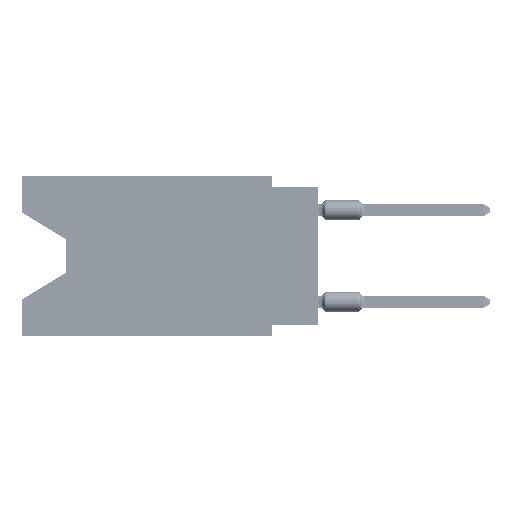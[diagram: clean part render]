
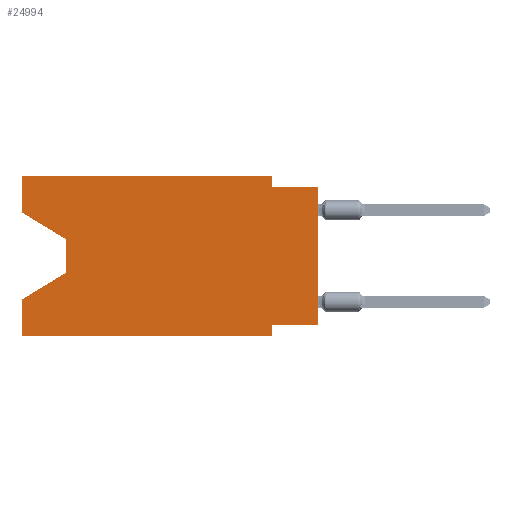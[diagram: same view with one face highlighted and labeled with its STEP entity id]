
A CAD part, left-side view. The second image highlights one B-rep face of the part: STEP entity #24994.
In plain terms, the highlighted planar face has unit normal (-1, 0, 0).
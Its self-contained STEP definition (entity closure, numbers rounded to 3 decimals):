
#139 = LINE ( 'NONE', #114180, #81911 ) ;
#1110 = EDGE_CURVE ( 'NONE', #107210, #41197, #100415, .T. ) ;
#3714 = DIRECTION ( 'NONE',  ( 0., 0.855, -0.519 ) ) ;
#4811 = CARTESIAN_POINT ( 'NONE',  ( 0., 16.383, 0. ) ) ;
#5050 = EDGE_LOOP ( 'NONE', ( #55344, #67228, #28012, #42846, #88379, #29049, #16364, #54764, #113163, #54858, #100345, #48149 ) ) ;
#8114 = CARTESIAN_POINT ( 'NONE',  ( 0., 13.97, -3.505 ) ) ;
#8500 = CARTESIAN_POINT ( 'NONE',  ( 0., 16.383, 0. ) ) ;
#9137 = VECTOR ( 'NONE', #3714, 1000. ) ;
#10500 = VERTEX_POINT ( 'NONE', #104164 ) ;
#11491 = EDGE_CURVE ( 'NONE', #29084, #54442, #13577, .T. ) ;
#11875 = LINE ( 'NONE', #30008, #97295 ) ;
#12349 = CARTESIAN_POINT ( 'NONE',  ( 0., 16.383, 0. ) ) ;
#12942 = CARTESIAN_POINT ( 'NONE',  ( 0., 13.97, -3.505 ) ) ;
#13577 = LINE ( 'NONE', #56252, #45236 ) ;
#14923 = CARTESIAN_POINT ( 'NONE',  ( 0., 16.383, -6.852 ) ) ;
#15691 = CARTESIAN_POINT ( 'NONE',  ( 0., 0., -8.255 ) ) ;
#16031 = VECTOR ( 'NONE', #113544, 1000. ) ;
#16187 = VERTEX_POINT ( 'NONE', #26955 ) ;
#16364 = ORIENTED_EDGE ( 'NONE', *, *, #80838, .F. ) ;
#17257 = EDGE_CURVE ( 'NONE', #10500, #16187, #61457, .T. ) ;
#18550 = VECTOR ( 'NONE', #60354, 1000. ) ;
#19495 = VECTOR ( 'NONE', #22275, 1000. ) ;
#20193 = FACE_OUTER_BOUND ( 'NONE', #5050, .T. ) ;
#20897 = CARTESIAN_POINT ( 'NONE',  ( 0., 16.383, -2.038 ) ) ;
#22275 = DIRECTION ( 'NONE',  ( 0., 0., 1. ) ) ;
#24994 = ADVANCED_FACE ( 'NONE', ( #20193 ), #84902, .F. ) ;
#25699 = VERTEX_POINT ( 'NONE', #15691 ) ;
#25888 = LINE ( 'NONE', #114182, #18550 ) ;
#26062 = LINE ( 'NONE', #8500, #71892 ) ;
#26821 = CARTESIAN_POINT ( 'NONE',  ( 0., 13.97, -5.385 ) ) ;
#26955 = CARTESIAN_POINT ( 'NONE',  ( 0., 2.54, -0.635 ) ) ;
#28012 = ORIENTED_EDGE ( 'NONE', *, *, #89920, .T. ) ;
#29049 = ORIENTED_EDGE ( 'NONE', *, *, #91329, .F. ) ;
#29084 = VERTEX_POINT ( 'NONE', #59069 ) ;
#30008 = CARTESIAN_POINT ( 'NONE',  ( 0., 0., -8.255 ) ) ;
#30489 = LINE ( 'NONE', #12349, #19495 ) ;
#31636 = LINE ( 'NONE', #111734, #78249 ) ;
#31715 = DIRECTION ( 'NONE',  ( 0., -1., 0. ) ) ;
#32287 = DIRECTION ( 'NONE',  ( 0., 0., -1. ) ) ;
#32775 = DIRECTION ( 'NONE',  ( 0., 0., 1. ) ) ;
#35383 = DIRECTION ( 'NONE',  ( 0., -1., 0. ) ) ;
#35418 = VECTOR ( 'NONE', #42100, 1000. ) ;
#35787 = DIRECTION ( 'NONE',  ( 0., 0., -1. ) ) ;
#35886 = VERTEX_POINT ( 'NONE', #73316 ) ;
#38751 = DIRECTION ( 'NONE',  ( 0., 1., 0. ) ) ;
#41197 = VERTEX_POINT ( 'NONE', #12942 ) ;
#42100 = DIRECTION ( 'NONE',  ( 0., -1., 0. ) ) ;
#42197 = CARTESIAN_POINT ( 'NONE',  ( 0., 2.54, 0. ) ) ;
#42846 = ORIENTED_EDGE ( 'NONE', *, *, #70744, .F. ) ;
#45236 = VECTOR ( 'NONE', #31715, 1000. ) ;
#48149 = ORIENTED_EDGE ( 'NONE', *, *, #78476, .F. ) ;
#51134 = CARTESIAN_POINT ( 'NONE',  ( 0., 16.383, 0. ) ) ;
#51431 = LINE ( 'NONE', #87700, #35418 ) ;
#51516 = DIRECTION ( 'NONE',  ( 1., 0., 0. ) ) ;
#54442 = VERTEX_POINT ( 'NONE', #76331 ) ;
#54764 = ORIENTED_EDGE ( 'NONE', *, *, #61824, .T. ) ;
#54858 = ORIENTED_EDGE ( 'NONE', *, *, #17257, .F. ) ;
#55344 = ORIENTED_EDGE ( 'NONE', *, *, #1110, .T. ) ;
#55789 = EDGE_CURVE ( 'NONE', #72220, #10500, #26062, .T. ) ;
#56252 = CARTESIAN_POINT ( 'NONE',  ( 0., 16.383, -8.89 ) ) ;
#59069 = CARTESIAN_POINT ( 'NONE',  ( 0., 16.383, -8.89 ) ) ;
#60354 = DIRECTION ( 'NONE',  ( 0., 0., 1. ) ) ;
#61457 = LINE ( 'NONE', #42197, #16031 ) ;
#61824 = EDGE_CURVE ( 'NONE', #25699, #35886, #25888, .T. ) ;
#64222 = VECTOR ( 'NONE', #115104, 1000. ) ;
#64727 = DIRECTION ( 'NONE',  ( 0., -0.855, -0.519 ) ) ;
#66817 = LINE ( 'NONE', #92572, #9137 ) ;
#67228 = ORIENTED_EDGE ( 'NONE', *, *, #101912, .T. ) ;
#67955 = CARTESIAN_POINT ( 'NONE',  ( 0., 16.383, -2.038 ) ) ;
#70744 = EDGE_CURVE ( 'NONE', #29084, #108419, #31636, .T. ) ;
#71892 = VECTOR ( 'NONE', #35383, 1000. ) ;
#72220 = VERTEX_POINT ( 'NONE', #51134 ) ;
#73077 = EDGE_CURVE ( 'NONE', #16187, #35886, #51431, .T. ) ;
#73316 = CARTESIAN_POINT ( 'NONE',  ( 0., 0., -0.635 ) ) ;
#73793 = VECTOR ( 'NONE', #64727, 1000. ) ;
#76331 = CARTESIAN_POINT ( 'NONE',  ( 0., 2.54, -8.89 ) ) ;
#78249 = VECTOR ( 'NONE', #32775, 1000. ) ;
#78476 = EDGE_CURVE ( 'NONE', #107210, #72220, #30489, .T. ) ;
#80838 = EDGE_CURVE ( 'NONE', #25699, #95341, #11875, .T. ) ;
#81911 = VECTOR ( 'NONE', #35787, 1000. ) ;
#84902 = PLANE ( 'NONE',  #106327 ) ;
#87700 = CARTESIAN_POINT ( 'NONE',  ( 0., 0., -0.635 ) ) ;
#88379 = ORIENTED_EDGE ( 'NONE', *, *, #11491, .T. ) ;
#89920 = EDGE_CURVE ( 'NONE', #102997, #108419, #66817, .T. ) ;
#91329 = EDGE_CURVE ( 'NONE', #95341, #54442, #139, .T. ) ;
#92572 = CARTESIAN_POINT ( 'NONE',  ( 0., 13.97, -5.385 ) ) ;
#95341 = VERTEX_POINT ( 'NONE', #114263 ) ;
#97295 = VECTOR ( 'NONE', #38751, 1000. ) ;
#100345 = ORIENTED_EDGE ( 'NONE', *, *, #55789, .F. ) ;
#100415 = LINE ( 'NONE', #20897, #73793 ) ;
#101912 = EDGE_CURVE ( 'NONE', #41197, #102997, #106324, .T. ) ;
#102997 = VERTEX_POINT ( 'NONE', #26821 ) ;
#104164 = CARTESIAN_POINT ( 'NONE',  ( 0., 2.54, 0. ) ) ;
#106324 = LINE ( 'NONE', #8114, #64222 ) ;
#106327 = AXIS2_PLACEMENT_3D ( 'NONE', #4811, #51516, #32287 ) ;
#107210 = VERTEX_POINT ( 'NONE', #67955 ) ;
#108419 = VERTEX_POINT ( 'NONE', #14923 ) ;
#111734 = CARTESIAN_POINT ( 'NONE',  ( 0., 16.383, 0. ) ) ;
#113163 = ORIENTED_EDGE ( 'NONE', *, *, #73077, .F. ) ;
#113544 = DIRECTION ( 'NONE',  ( 0., 0., -1. ) ) ;
#114180 = CARTESIAN_POINT ( 'NONE',  ( 0., 2.54, -8.89 ) ) ;
#114182 = CARTESIAN_POINT ( 'NONE',  ( 0., 0., 0. ) ) ;
#114263 = CARTESIAN_POINT ( 'NONE',  ( 0., 2.54, -8.255 ) ) ;
#115104 = DIRECTION ( 'NONE',  ( 0., 0., -1. ) ) ;
